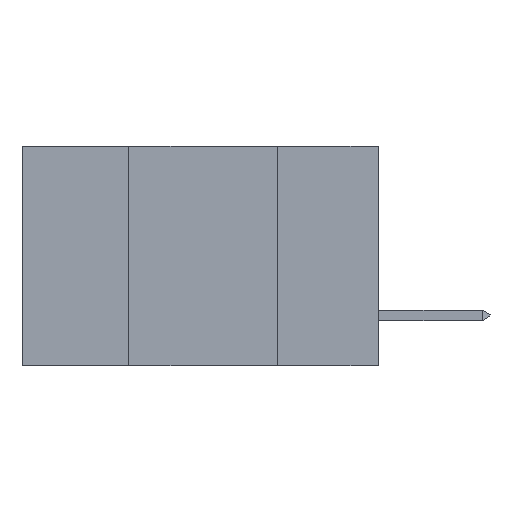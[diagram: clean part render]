
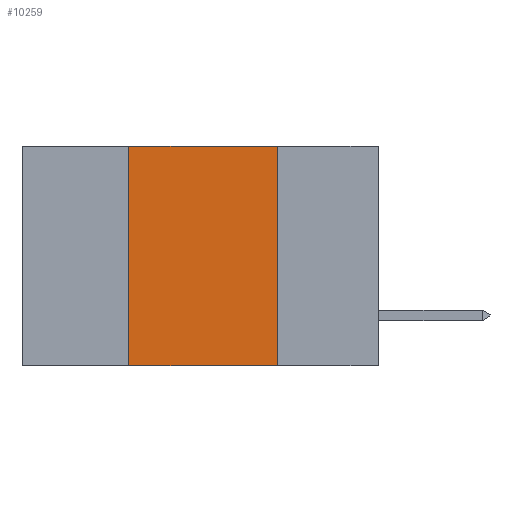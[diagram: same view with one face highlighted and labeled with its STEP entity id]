
A CAD part, left-side view. The second image highlights one B-rep face of the part: STEP entity #10259.
In plain terms, the highlighted planar face has unit normal (-1, 0, 0).
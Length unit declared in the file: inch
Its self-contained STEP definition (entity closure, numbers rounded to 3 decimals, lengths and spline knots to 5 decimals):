
#139 = CARTESIAN_POINT ( 'NONE',  ( 0., 0.17, -0.37 ) ) ;
#1045 = CARTESIAN_POINT ( 'NONE',  ( 0., 0.6, -0.37 ) ) ;
#1114 = LINE ( 'NONE', #1045, #7134 ) ;
#2045 = ORIENTED_EDGE ( 'NONE', *, *, #2817, .F. ) ;
#2249 = DIRECTION ( 'NONE',  ( 0., 0., 1. ) ) ;
#2387 = VECTOR ( 'NONE', #2249, 39.37008 ) ;
#2817 = EDGE_CURVE ( 'NONE', #9766, #5004, #12915, .T. ) ;
#2920 = EDGE_CURVE ( 'NONE', #6974, #9766, #2965, .T. ) ;
#2965 = LINE ( 'NONE', #11025, #6580 ) ;
#3953 = EDGE_CURVE ( 'NONE', #5218, #6974, #4212, .T. ) ;
#4212 = LINE ( 'NONE', #7675, #2387 ) ;
#4337 = PLANE ( 'NONE',  #7702 ) ;
#4597 = CARTESIAN_POINT ( 'NONE',  ( 0., 0.42, -0.37 ) ) ;
#4611 = DIRECTION ( 'NONE',  ( 0., -1., 0. ) ) ;
#5004 = VERTEX_POINT ( 'NONE', #139 ) ;
#5218 = VERTEX_POINT ( 'NONE', #4597 ) ;
#6153 = EDGE_CURVE ( 'NONE', #5218, #5004, #1114, .T. ) ;
#6580 = VECTOR ( 'NONE', #11195, 39.37008 ) ;
#6585 = DIRECTION ( 'NONE',  ( 0., 0., -1. ) ) ;
#6974 = VERTEX_POINT ( 'NONE', #13010 ) ;
#7134 = VECTOR ( 'NONE', #4611, 39.37008 ) ;
#7272 = DIRECTION ( 'NONE',  ( 0., 0., -1. ) ) ;
#7571 = DIRECTION ( 'NONE',  ( 1., 0., 0. ) ) ;
#7644 = FACE_OUTER_BOUND ( 'NONE', #9834, .T. ) ;
#7675 = CARTESIAN_POINT ( 'NONE',  ( 0., 0.42, -0.37 ) ) ;
#7702 = AXIS2_PLACEMENT_3D ( 'NONE', #13343, #7571, #6585 ) ;
#9511 = ORIENTED_EDGE ( 'NONE', *, *, #6153, .T. ) ;
#9766 = VERTEX_POINT ( 'NONE', #9785 ) ;
#9785 = CARTESIAN_POINT ( 'NONE',  ( 0., 0.17, 0. ) ) ;
#9834 = EDGE_LOOP ( 'NONE', ( #2045, #12707, #11359, #9511 ) ) ;
#10259 = ADVANCED_FACE ( 'NONE', ( #7644 ), #4337, .F. ) ;
#11025 = CARTESIAN_POINT ( 'NONE',  ( 0., 0.6, 0. ) ) ;
#11195 = DIRECTION ( 'NONE',  ( 0., -1., 0. ) ) ;
#11359 = ORIENTED_EDGE ( 'NONE', *, *, #3953, .F. ) ;
#12707 = ORIENTED_EDGE ( 'NONE', *, *, #2920, .F. ) ;
#12915 = LINE ( 'NONE', #12991, #13999 ) ;
#12991 = CARTESIAN_POINT ( 'NONE',  ( 0., 0.17, -0.37 ) ) ;
#13010 = CARTESIAN_POINT ( 'NONE',  ( 0., 0.42, 0. ) ) ;
#13343 = CARTESIAN_POINT ( 'NONE',  ( 0., 0.6, 0. ) ) ;
#13999 = VECTOR ( 'NONE', #7272, 39.37008 ) ;
